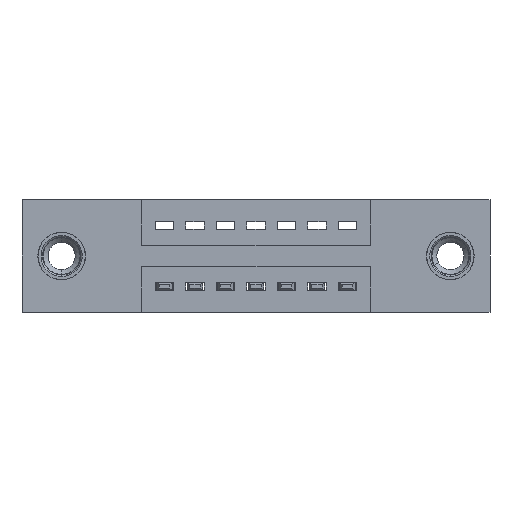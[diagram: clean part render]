
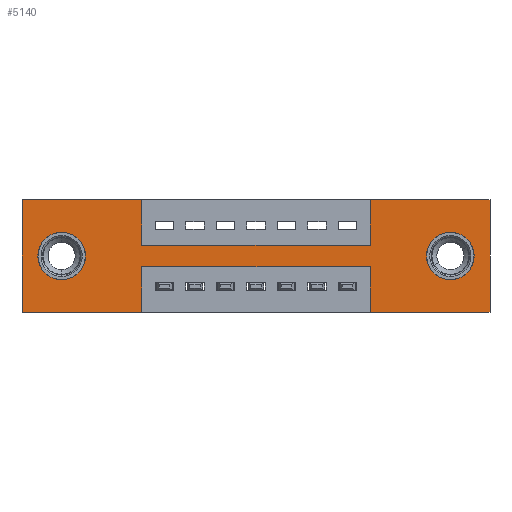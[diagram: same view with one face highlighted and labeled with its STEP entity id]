
A CAD part, front view. The second image highlights one B-rep face of the part: STEP entity #5140.
In plain terms, the highlighted planar face has unit normal (0, -1, 0).
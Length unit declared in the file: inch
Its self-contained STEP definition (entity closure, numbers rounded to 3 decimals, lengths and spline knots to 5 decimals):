
#148 = EDGE_CURVE ( 'NONE', #652, #854, #6317, .T. ) ;
#197 = CARTESIAN_POINT ( 'NONE',  ( 0.13, 0., -0.107 ) ) ;
#250 = LINE ( 'NONE', #10764, #7150 ) ;
#355 = CARTESIAN_POINT ( 'NONE',  ( 0., 0., -0.37 ) ) ;
#611 = CARTESIAN_POINT ( 'NONE',  ( 1.535, 0., -0.37 ) ) ;
#652 = VERTEX_POINT ( 'NONE', #4993 ) ;
#680 = EDGE_LOOP ( 'NONE', ( #2257, #10110 ) ) ;
#854 = VERTEX_POINT ( 'NONE', #4759 ) ;
#870 = DIRECTION ( 'NONE',  ( 0., 0., 1. ) ) ;
#1020 = VERTEX_POINT ( 'NONE', #6984 ) ;
#1100 = ORIENTED_EDGE ( 'NONE', *, *, #9467, .F. ) ;
#1126 = DIRECTION ( 'NONE',  ( 0., 1., 0. ) ) ;
#1140 = VERTEX_POINT ( 'NONE', #9220 ) ;
#1189 = CIRCLE ( 'NONE', #5679, 0.078 ) ;
#1492 = VECTOR ( 'NONE', #4334, 39.37008 ) ;
#1594 = CARTESIAN_POINT ( 'NONE',  ( 0.3925, 0., -0.22 ) ) ;
#1596 = ORIENTED_EDGE ( 'NONE', *, *, #7892, .F. ) ;
#1683 = LINE ( 'NONE', #3555, #6121 ) ;
#1699 = ORIENTED_EDGE ( 'NONE', *, *, #9746, .F. ) ;
#1712 = ORIENTED_EDGE ( 'NONE', *, *, #7553, .F. ) ;
#1752 = VECTOR ( 'NONE', #2979, 39.37008 ) ;
#1766 = CARTESIAN_POINT ( 'NONE',  ( 0., 0., -0.37 ) ) ;
#1845 = VERTEX_POINT ( 'NONE', #10691 ) ;
#2105 = CARTESIAN_POINT ( 'NONE',  ( 1.1425, 0., 0. ) ) ;
#2149 = LINE ( 'NONE', #10399, #6502 ) ;
#2257 = ORIENTED_EDGE ( 'NONE', *, *, #7937, .T. ) ;
#2414 = CARTESIAN_POINT ( 'NONE',  ( 0., 0., 0. ) ) ;
#2439 = FACE_BOUND ( 'NONE', #10323, .T. ) ;
#2448 = LINE ( 'NONE', #2676, #4620 ) ;
#2526 = VERTEX_POINT ( 'NONE', #2714 ) ;
#2603 = CARTESIAN_POINT ( 'NONE',  ( 0.13, 0., -0.263 ) ) ;
#2676 = CARTESIAN_POINT ( 'NONE',  ( 0., 0., 0. ) ) ;
#2714 = CARTESIAN_POINT ( 'NONE',  ( 0.3925, 0., -0.22 ) ) ;
#2938 = AXIS2_PLACEMENT_3D ( 'NONE', #6451, #1126, #7260 ) ;
#2979 = DIRECTION ( 'NONE',  ( 0., 0., 1. ) ) ;
#3100 = VECTOR ( 'NONE', #7665, 39.37008 ) ;
#3120 = EDGE_LOOP ( 'NONE', ( #6744, #1699, #6258, #7266, #1712, #4192, #1100, #6905, #5018, #8992, #1596, #10650 ) ) ;
#3322 = EDGE_CURVE ( 'NONE', #7577, #8636, #250, .T. ) ;
#3555 = CARTESIAN_POINT ( 'NONE',  ( 0.3925, 0., -0.15 ) ) ;
#3644 = LINE ( 'NONE', #1594, #8273 ) ;
#3658 = EDGE_CURVE ( 'NONE', #7232, #1140, #2149, .T. ) ;
#3749 = ORIENTED_EDGE ( 'NONE', *, *, #9922, .T. ) ;
#3843 = VERTEX_POINT ( 'NONE', #2603 ) ;
#4032 = CARTESIAN_POINT ( 'NONE',  ( 1.1425, 0., -0.15 ) ) ;
#4083 = DIRECTION ( 'NONE',  ( -1., 0., 0. ) ) ;
#4192 = ORIENTED_EDGE ( 'NONE', *, *, #5578, .F. ) ;
#4198 = EDGE_CURVE ( 'NONE', #5071, #7232, #7538, .T. ) ;
#4237 = LINE ( 'NONE', #5585, #1752 ) ;
#4279 = LINE ( 'NONE', #9881, #1492 ) ;
#4318 = LINE ( 'NONE', #2414, #10604 ) ;
#4334 = DIRECTION ( 'NONE',  ( 0., 0., 1. ) ) ;
#4346 = CIRCLE ( 'NONE', #7144, 0.078 ) ;
#4400 = DIRECTION ( 'NONE',  ( 0., 1., 0. ) ) ;
#4561 = DIRECTION ( 'NONE',  ( 0., 0., -1. ) ) ;
#4585 = ORIENTED_EDGE ( 'NONE', *, *, #5316, .T. ) ;
#4620 = VECTOR ( 'NONE', #8517, 39.37008 ) ;
#4730 = AXIS2_PLACEMENT_3D ( 'NONE', #9574, #4847, #10320 ) ;
#4739 = CIRCLE ( 'NONE', #2938, 0.078 ) ;
#4759 = CARTESIAN_POINT ( 'NONE',  ( 1.405, 0., -0.107 ) ) ;
#4819 = VERTEX_POINT ( 'NONE', #4032 ) ;
#4847 = DIRECTION ( 'NONE',  ( 0., 1., 0. ) ) ;
#4993 = CARTESIAN_POINT ( 'NONE',  ( 1.405, 0., -0.263 ) ) ;
#5018 = ORIENTED_EDGE ( 'NONE', *, *, #3322, .F. ) ;
#5071 = VERTEX_POINT ( 'NONE', #611 ) ;
#5140 = ADVANCED_FACE ( 'NONE', ( #9806, #2439, #6763 ), #10013, .T. ) ;
#5294 = DIRECTION ( 'NONE',  ( 1., 0., 0. ) ) ;
#5316 = EDGE_CURVE ( 'NONE', #3843, #5429, #4739, .T. ) ;
#5391 = VECTOR ( 'NONE', #4083, 39.37008 ) ;
#5429 = VERTEX_POINT ( 'NONE', #197 ) ;
#5436 = LINE ( 'NONE', #6069, #3100 ) ;
#5491 = DIRECTION ( 'NONE',  ( 0., 0., -1. ) ) ;
#5578 = EDGE_CURVE ( 'NONE', #8258, #8571, #4318, .T. ) ;
#5585 = CARTESIAN_POINT ( 'NONE',  ( 1.1425, 0., 0. ) ) ;
#5679 = AXIS2_PLACEMENT_3D ( 'NONE', #9180, #4400, #9954 ) ;
#5705 = LINE ( 'NONE', #10196, #7589 ) ;
#5734 = DIRECTION ( 'NONE',  ( 0., 0., 1. ) ) ;
#6069 = CARTESIAN_POINT ( 'NONE',  ( 0., 0., -0.37 ) ) ;
#6121 = VECTOR ( 'NONE', #5294, 39.37008 ) ;
#6191 = DIRECTION ( 'NONE',  ( 0., 0., -1. ) ) ;
#6258 = ORIENTED_EDGE ( 'NONE', *, *, #3658, .F. ) ;
#6271 = DIRECTION ( 'NONE',  ( 0., 1., 0. ) ) ;
#6317 = CIRCLE ( 'NONE', #4730, 0.078 ) ;
#6451 = CARTESIAN_POINT ( 'NONE',  ( 0.13, 0., -0.185 ) ) ;
#6502 = VECTOR ( 'NONE', #5734, 39.37008 ) ;
#6712 = VERTEX_POINT ( 'NONE', #355 ) ;
#6744 = ORIENTED_EDGE ( 'NONE', *, *, #8660, .F. ) ;
#6763 = FACE_OUTER_BOUND ( 'NONE', #3120, .T. ) ;
#6872 = EDGE_CURVE ( 'NONE', #8636, #4819, #1683, .T. ) ;
#6905 = ORIENTED_EDGE ( 'NONE', *, *, #6872, .F. ) ;
#6984 = CARTESIAN_POINT ( 'NONE',  ( 0.3925, 0., -0.37 ) ) ;
#7144 = AXIS2_PLACEMENT_3D ( 'NONE', #10883, #6271, #870 ) ;
#7150 = VECTOR ( 'NONE', #10795, 39.37008 ) ;
#7232 = VERTEX_POINT ( 'NONE', #9805 ) ;
#7260 = DIRECTION ( 'NONE',  ( 0., 0., 1. ) ) ;
#7266 = ORIENTED_EDGE ( 'NONE', *, *, #4198, .F. ) ;
#7538 = LINE ( 'NONE', #8903, #5391 ) ;
#7553 = EDGE_CURVE ( 'NONE', #8571, #5071, #5705, .T. ) ;
#7577 = VERTEX_POINT ( 'NONE', #9454 ) ;
#7589 = VECTOR ( 'NONE', #5491, 39.37008 ) ;
#7631 = DIRECTION ( 'NONE',  ( -1., 0., 0. ) ) ;
#7665 = DIRECTION ( 'NONE',  ( -1., 0., 0. ) ) ;
#7684 = AXIS2_PLACEMENT_3D ( 'NONE', #1766, #9319, #4561 ) ;
#7892 = EDGE_CURVE ( 'NONE', #6712, #1845, #4279, .T. ) ;
#7937 = EDGE_CURVE ( 'NONE', #854, #652, #1189, .T. ) ;
#7966 = EDGE_CURVE ( 'NONE', #1020, #6712, #5436, .T. ) ;
#8258 = VERTEX_POINT ( 'NONE', #2105 ) ;
#8273 = VECTOR ( 'NONE', #7631, 39.37008 ) ;
#8517 = DIRECTION ( 'NONE',  ( 1., 0., 0. ) ) ;
#8571 = VERTEX_POINT ( 'NONE', #9200 ) ;
#8636 = VERTEX_POINT ( 'NONE', #10028 ) ;
#8660 = EDGE_CURVE ( 'NONE', #2526, #1020, #8781, .T. ) ;
#8781 = LINE ( 'NONE', #9300, #10312 ) ;
#8903 = CARTESIAN_POINT ( 'NONE',  ( 0., 0., -0.37 ) ) ;
#8992 = ORIENTED_EDGE ( 'NONE', *, *, #9867, .F. ) ;
#9084 = DIRECTION ( 'NONE',  ( 1., 0., 0. ) ) ;
#9180 = CARTESIAN_POINT ( 'NONE',  ( 1.405, 0., -0.185 ) ) ;
#9200 = CARTESIAN_POINT ( 'NONE',  ( 1.535, 0., 0. ) ) ;
#9220 = CARTESIAN_POINT ( 'NONE',  ( 1.1425, 0., -0.22 ) ) ;
#9300 = CARTESIAN_POINT ( 'NONE',  ( 0.3925, 0., -0.37 ) ) ;
#9319 = DIRECTION ( 'NONE',  ( 0., -1., 0. ) ) ;
#9454 = CARTESIAN_POINT ( 'NONE',  ( 0.3925, 0., 0. ) ) ;
#9467 = EDGE_CURVE ( 'NONE', #4819, #8258, #4237, .T. ) ;
#9574 = CARTESIAN_POINT ( 'NONE',  ( 1.405, 0., -0.185 ) ) ;
#9746 = EDGE_CURVE ( 'NONE', #1140, #2526, #3644, .T. ) ;
#9805 = CARTESIAN_POINT ( 'NONE',  ( 1.1425, 0., -0.37 ) ) ;
#9806 = FACE_BOUND ( 'NONE', #680, .T. ) ;
#9867 = EDGE_CURVE ( 'NONE', #1845, #7577, #2448, .T. ) ;
#9881 = CARTESIAN_POINT ( 'NONE',  ( 0., 0., 0. ) ) ;
#9922 = EDGE_CURVE ( 'NONE', #5429, #3843, #4346, .T. ) ;
#9954 = DIRECTION ( 'NONE',  ( 0., 0., -1. ) ) ;
#10013 = PLANE ( 'NONE',  #7684 ) ;
#10028 = CARTESIAN_POINT ( 'NONE',  ( 0.3925, 0., -0.15 ) ) ;
#10110 = ORIENTED_EDGE ( 'NONE', *, *, #148, .T. ) ;
#10196 = CARTESIAN_POINT ( 'NONE',  ( 1.535, 0., 0. ) ) ;
#10312 = VECTOR ( 'NONE', #6191, 39.37008 ) ;
#10320 = DIRECTION ( 'NONE',  ( 0., 0., -1. ) ) ;
#10323 = EDGE_LOOP ( 'NONE', ( #3749, #4585 ) ) ;
#10399 = CARTESIAN_POINT ( 'NONE',  ( 1.1425, 0., -0.37 ) ) ;
#10604 = VECTOR ( 'NONE', #9084, 39.37008 ) ;
#10650 = ORIENTED_EDGE ( 'NONE', *, *, #7966, .F. ) ;
#10691 = CARTESIAN_POINT ( 'NONE',  ( 0., 0., 0. ) ) ;
#10764 = CARTESIAN_POINT ( 'NONE',  ( 0.3925, 0., 0. ) ) ;
#10795 = DIRECTION ( 'NONE',  ( 0., 0., -1. ) ) ;
#10883 = CARTESIAN_POINT ( 'NONE',  ( 0.13, 0., -0.185 ) ) ;
